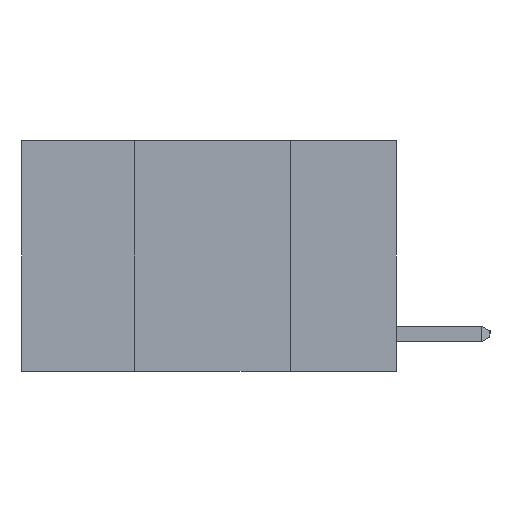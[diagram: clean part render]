
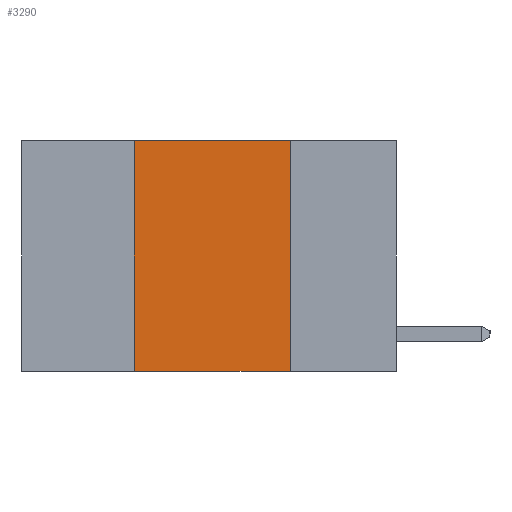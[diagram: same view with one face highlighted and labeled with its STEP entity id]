
A CAD part, left-side view. The second image highlights one B-rep face of the part: STEP entity #3290.
In plain terms, the highlighted planar face has unit normal (-1, 0, 0).
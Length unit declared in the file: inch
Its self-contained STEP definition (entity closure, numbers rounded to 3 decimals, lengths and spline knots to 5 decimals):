
#623 = VERTEX_POINT ( 'NONE', #2698 ) ;
#1190 = VERTEX_POINT ( 'NONE', #1816 ) ;
#1389 = CARTESIAN_POINT ( 'NONE',  ( 0., 0.6, -0.37 ) ) ;
#1816 = CARTESIAN_POINT ( 'NONE',  ( 0., 0.42, 0. ) ) ;
#2333 = PLANE ( 'NONE',  #4222 ) ;
#2419 = VECTOR ( 'NONE', #11665, 39.37008 ) ;
#2626 = ORIENTED_EDGE ( 'NONE', *, *, #6181, .T. ) ;
#2698 = CARTESIAN_POINT ( 'NONE',  ( 0., 0.17, 0. ) ) ;
#3290 = ADVANCED_FACE ( 'NONE', ( #4150 ), #2333, .F. ) ;
#3474 = VECTOR ( 'NONE', #12782, 39.37008 ) ;
#3653 = DIRECTION ( 'NONE',  ( 0., 0., -1. ) ) ;
#4150 = FACE_OUTER_BOUND ( 'NONE', #4537, .T. ) ;
#4222 = AXIS2_PLACEMENT_3D ( 'NONE', #6207, #11288, #3653 ) ;
#4537 = EDGE_LOOP ( 'NONE', ( #8302, #8686, #12393, #2626 ) ) ;
#5885 = EDGE_CURVE ( 'NONE', #12597, #1190, #6908, .T. ) ;
#6181 = EDGE_CURVE ( 'NONE', #12597, #8563, #6290, .T. ) ;
#6207 = CARTESIAN_POINT ( 'NONE',  ( 0., 0.6, 0. ) ) ;
#6290 = LINE ( 'NONE', #1389, #2419 ) ;
#6908 = LINE ( 'NONE', #11490, #3474 ) ;
#7701 = CARTESIAN_POINT ( 'NONE',  ( 0., 0.17, -0.37 ) ) ;
#8005 = LINE ( 'NONE', #16228, #11741 ) ;
#8302 = ORIENTED_EDGE ( 'NONE', *, *, #8459, .F. ) ;
#8459 = EDGE_CURVE ( 'NONE', #623, #8563, #8005, .T. ) ;
#8515 = EDGE_CURVE ( 'NONE', #1190, #623, #10959, .T. ) ;
#8563 = VERTEX_POINT ( 'NONE', #7701 ) ;
#8686 = ORIENTED_EDGE ( 'NONE', *, *, #8515, .F. ) ;
#8797 = CARTESIAN_POINT ( 'NONE',  ( 0., 0.6, 0. ) ) ;
#10124 = DIRECTION ( 'NONE',  ( 0., -1., 0. ) ) ;
#10756 = CARTESIAN_POINT ( 'NONE',  ( 0., 0.42, -0.37 ) ) ;
#10959 = LINE ( 'NONE', #8797, #13840 ) ;
#11266 = DIRECTION ( 'NONE',  ( 0., 0., -1. ) ) ;
#11288 = DIRECTION ( 'NONE',  ( 1., 0., 0. ) ) ;
#11490 = CARTESIAN_POINT ( 'NONE',  ( 0., 0.42, 0. ) ) ;
#11665 = DIRECTION ( 'NONE',  ( 0., -1., 0. ) ) ;
#11741 = VECTOR ( 'NONE', #11266, 39.37008 ) ;
#12393 = ORIENTED_EDGE ( 'NONE', *, *, #5885, .F. ) ;
#12597 = VERTEX_POINT ( 'NONE', #10756 ) ;
#12782 = DIRECTION ( 'NONE',  ( 0., 0., 1. ) ) ;
#13840 = VECTOR ( 'NONE', #10124, 39.37008 ) ;
#16228 = CARTESIAN_POINT ( 'NONE',  ( 0., 0.17, 0. ) ) ;
